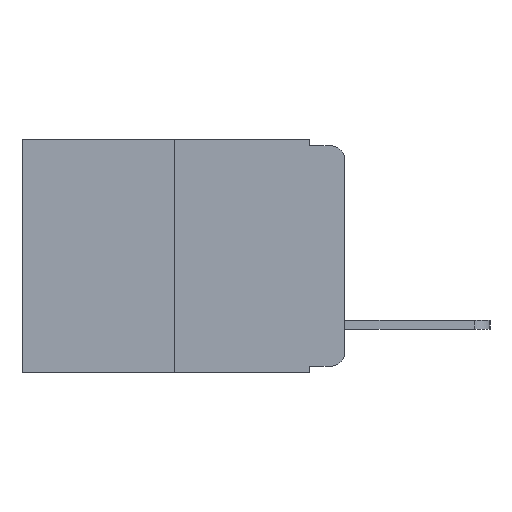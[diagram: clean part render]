
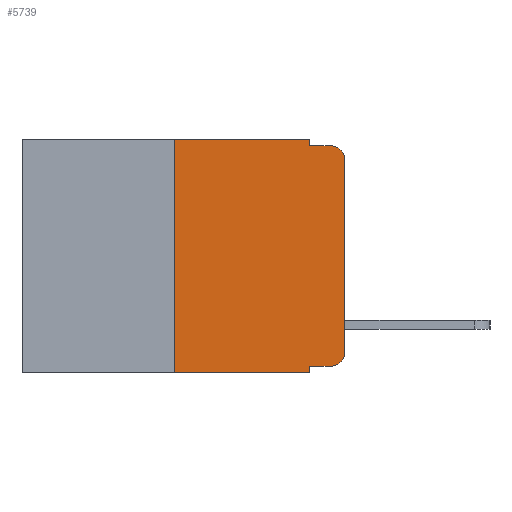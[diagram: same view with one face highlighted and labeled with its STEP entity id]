
A CAD part, left-side view. The second image highlights one B-rep face of the part: STEP entity #5739.
In plain terms, the highlighted planar face has unit normal (-1, 0, 0).
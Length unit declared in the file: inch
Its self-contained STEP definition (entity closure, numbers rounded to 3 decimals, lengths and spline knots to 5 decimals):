
#367 = LINE ( 'NONE', #6583, #12990 ) ;
#654 = ORIENTED_EDGE ( 'NONE', *, *, #7844, .T. ) ;
#822 = EDGE_LOOP ( 'NONE', ( #654, #7691, #4745, #8075, #13761, #11798, #14350, #2475, #12136, #14602 ) ) ;
#956 = VERTEX_POINT ( 'NONE', #2457 ) ;
#1091 = VERTEX_POINT ( 'NONE', #12334 ) ;
#1350 = FACE_OUTER_BOUND ( 'NONE', #822, .T. ) ;
#1434 = VERTEX_POINT ( 'NONE', #14764 ) ;
#2110 = AXIS2_PLACEMENT_3D ( 'NONE', #3308, #3553, #3516 ) ;
#2334 = VERTEX_POINT ( 'NONE', #6082 ) ;
#2457 = CARTESIAN_POINT ( 'NONE',  ( 0., 0.051, 0. ) ) ;
#2475 = ORIENTED_EDGE ( 'NONE', *, *, #8048, .F. ) ;
#3025 = VECTOR ( 'NONE', #7192, 39.37008 ) ;
#3196 = CARTESIAN_POINT ( 'NONE',  ( 0., 0.25, -0.343 ) ) ;
#3259 = CARTESIAN_POINT ( 'NONE',  ( 0., 0.02, -0.313 ) ) ;
#3308 = CARTESIAN_POINT ( 'NONE',  ( 0., 0.473, 0. ) ) ;
#3455 = VECTOR ( 'NONE', #4987, 39.37008 ) ;
#3516 = DIRECTION ( 'NONE',  ( 0., 0., -1. ) ) ;
#3553 = DIRECTION ( 'NONE',  ( 1., 0., 0. ) ) ;
#3559 = DIRECTION ( 'NONE',  ( 0., 0., 1. ) ) ;
#3681 = LINE ( 'NONE', #11395, #6651 ) ;
#4117 = CARTESIAN_POINT ( 'NONE',  ( 0., 0.051, 0. ) ) ;
#4281 = VERTEX_POINT ( 'NONE', #3196 ) ;
#4380 = PLANE ( 'NONE',  #2110 ) ;
#4515 = CARTESIAN_POINT ( 'NONE',  ( 0., 0.02, -0.01 ) ) ;
#4745 = ORIENTED_EDGE ( 'NONE', *, *, #7875, .F. ) ;
#4908 = DIRECTION ( 'NONE',  ( 0., 0., -1. ) ) ;
#4947 = DIRECTION ( 'NONE',  ( -1., 0., 0. ) ) ;
#4984 = DIRECTION ( 'NONE',  ( 0., -1., 0. ) ) ;
#4987 = DIRECTION ( 'NONE',  ( 0., 0., -1. ) ) ;
#5335 = CARTESIAN_POINT ( 'NONE',  ( 0., 0.473, -0.343 ) ) ;
#5739 = ADVANCED_FACE ( 'NONE', ( #1350 ), #4380, .F. ) ;
#6082 = CARTESIAN_POINT ( 'NONE',  ( 0., 0., -0.313 ) ) ;
#6156 = AXIS2_PLACEMENT_3D ( 'NONE', #3259, #4947, #4908 ) ;
#6194 = VERTEX_POINT ( 'NONE', #8709 ) ;
#6272 = VECTOR ( 'NONE', #4984, 39.37008 ) ;
#6427 = LINE ( 'NONE', #12876, #12230 ) ;
#6583 = CARTESIAN_POINT ( 'NONE',  ( 0., 0.473, 0. ) ) ;
#6626 = VERTEX_POINT ( 'NONE', #4515 ) ;
#6651 = VECTOR ( 'NONE', #14171, 39.37008 ) ;
#6833 = LINE ( 'NONE', #4117, #3455 ) ;
#7031 = AXIS2_PLACEMENT_3D ( 'NONE', #8984, #7954, #8332 ) ;
#7192 = DIRECTION ( 'NONE',  ( 0., 0., -1. ) ) ;
#7228 = EDGE_CURVE ( 'NONE', #4281, #1434, #9453, .T. ) ;
#7500 = EDGE_CURVE ( 'NONE', #14918, #956, #367, .T. ) ;
#7691 = ORIENTED_EDGE ( 'NONE', *, *, #8046, .T. ) ;
#7798 = VERTEX_POINT ( 'NONE', #14403 ) ;
#7844 = EDGE_CURVE ( 'NONE', #2334, #6194, #13856, .T. ) ;
#7875 = EDGE_CURVE ( 'NONE', #7798, #6626, #3681, .T. ) ;
#7954 = DIRECTION ( 'NONE',  ( -1., 0., 0. ) ) ;
#8033 = EDGE_CURVE ( 'NONE', #1091, #2334, #13127, .T. ) ;
#8046 = EDGE_CURVE ( 'NONE', #6194, #6626, #10327, .T. ) ;
#8048 = EDGE_CURVE ( 'NONE', #10859, #1434, #6833, .T. ) ;
#8053 = EDGE_CURVE ( 'NONE', #10859, #1091, #9943, .T. ) ;
#8073 = EDGE_CURVE ( 'NONE', #956, #7798, #12533, .T. ) ;
#8075 = ORIENTED_EDGE ( 'NONE', *, *, #8073, .F. ) ;
#8076 = EDGE_CURVE ( 'NONE', #4281, #14918, #6427, .T. ) ;
#8272 = CARTESIAN_POINT ( 'NONE',  ( 0., 0.051, -0.333 ) ) ;
#8316 = CARTESIAN_POINT ( 'NONE',  ( 0., 0.25, 0. ) ) ;
#8332 = DIRECTION ( 'NONE',  ( 0., 0., -1. ) ) ;
#8599 = DIRECTION ( 'NONE',  ( 0., -1., 0. ) ) ;
#8709 = CARTESIAN_POINT ( 'NONE',  ( 0., 0., -0.03 ) ) ;
#8984 = CARTESIAN_POINT ( 'NONE',  ( 0., 0.02, -0.03 ) ) ;
#9453 = LINE ( 'NONE', #5335, #6272 ) ;
#9592 = VECTOR ( 'NONE', #11334, 39.37008 ) ;
#9626 = CARTESIAN_POINT ( 'NONE',  ( 0., 0., 0. ) ) ;
#9943 = LINE ( 'NONE', #8272, #9592 ) ;
#10327 = CIRCLE ( 'NONE', #7031, 0.02 ) ;
#10502 = VECTOR ( 'NONE', #11977, 39.37008 ) ;
#10859 = VERTEX_POINT ( 'NONE', #11672 ) ;
#11334 = DIRECTION ( 'NONE',  ( 0., -1., 0. ) ) ;
#11395 = CARTESIAN_POINT ( 'NONE',  ( 0., 0.051, -0.01 ) ) ;
#11672 = CARTESIAN_POINT ( 'NONE',  ( 0., 0.051, -0.333 ) ) ;
#11798 = ORIENTED_EDGE ( 'NONE', *, *, #8076, .F. ) ;
#11977 = DIRECTION ( 'NONE',  ( 0., 0., 1. ) ) ;
#12136 = ORIENTED_EDGE ( 'NONE', *, *, #8053, .T. ) ;
#12230 = VECTOR ( 'NONE', #3559, 39.37008 ) ;
#12334 = CARTESIAN_POINT ( 'NONE',  ( 0., 0.02, -0.333 ) ) ;
#12533 = LINE ( 'NONE', #13696, #3025 ) ;
#12876 = CARTESIAN_POINT ( 'NONE',  ( 0., 0.25, 0. ) ) ;
#12990 = VECTOR ( 'NONE', #8599, 39.37008 ) ;
#13127 = CIRCLE ( 'NONE', #6156, 0.02 ) ;
#13696 = CARTESIAN_POINT ( 'NONE',  ( 0., 0.051, 0. ) ) ;
#13761 = ORIENTED_EDGE ( 'NONE', *, *, #7500, .F. ) ;
#13856 = LINE ( 'NONE', #9626, #10502 ) ;
#14171 = DIRECTION ( 'NONE',  ( 0., -1., 0. ) ) ;
#14350 = ORIENTED_EDGE ( 'NONE', *, *, #7228, .T. ) ;
#14403 = CARTESIAN_POINT ( 'NONE',  ( 0., 0.051, -0.01 ) ) ;
#14602 = ORIENTED_EDGE ( 'NONE', *, *, #8033, .T. ) ;
#14764 = CARTESIAN_POINT ( 'NONE',  ( 0., 0.051, -0.343 ) ) ;
#14918 = VERTEX_POINT ( 'NONE', #8316 ) ;
